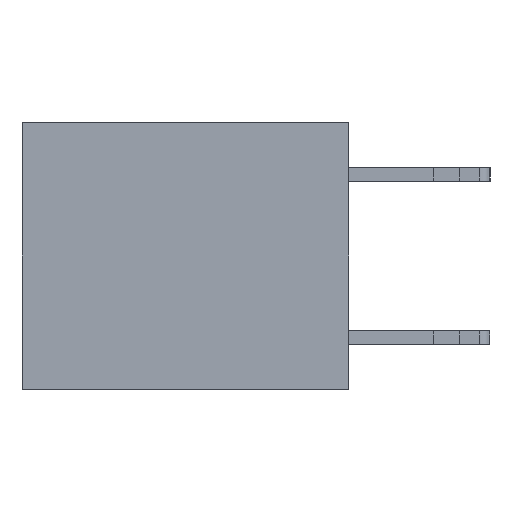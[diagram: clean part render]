
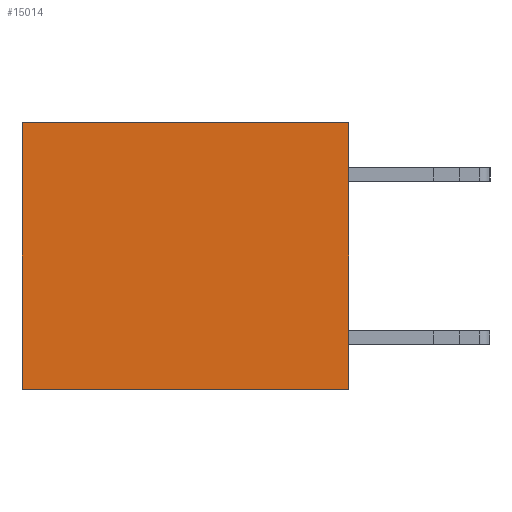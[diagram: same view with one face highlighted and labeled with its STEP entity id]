
A CAD part, left-side view. The second image highlights one B-rep face of the part: STEP entity #15014.
In plain terms, the highlighted planar face has unit normal (-1, 0, 0).
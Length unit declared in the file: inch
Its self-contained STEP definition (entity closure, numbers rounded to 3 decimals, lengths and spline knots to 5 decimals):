
#564 = EDGE_CURVE ( 'NONE', #7860, #4236, #18964, .T. ) ;
#1781 = VECTOR ( 'NONE', #2009, 39.37008 ) ;
#2009 = DIRECTION ( 'NONE',  ( 0., 0., -1. ) ) ;
#2299 = ORIENTED_EDGE ( 'NONE', *, *, #19089, .F. ) ;
#3406 = CARTESIAN_POINT ( 'NONE',  ( 0.3165, 0., 0. ) ) ;
#3525 = CARTESIAN_POINT ( 'NONE',  ( 0.3165, 0., -0.49 ) ) ;
#4236 = VERTEX_POINT ( 'NONE', #15485 ) ;
#5032 = DIRECTION ( 'NONE',  ( 0., 1., 0. ) ) ;
#5411 = CARTESIAN_POINT ( 'NONE',  ( 0.3165, 0., -0.49 ) ) ;
#6189 = VERTEX_POINT ( 'NONE', #16741 ) ;
#6247 = ORIENTED_EDGE ( 'NONE', *, *, #11554, .T. ) ;
#6881 = CARTESIAN_POINT ( 'NONE',  ( 0.3165, 0., -0.49 ) ) ;
#7126 = VERTEX_POINT ( 'NONE', #14093 ) ;
#7707 = LINE ( 'NONE', #3406, #12922 ) ;
#7860 = VERTEX_POINT ( 'NONE', #13289 ) ;
#8170 = VECTOR ( 'NONE', #17472, 39.37008 ) ;
#10008 = DIRECTION ( 'NONE',  ( 1., 0., 0. ) ) ;
#11113 = FACE_OUTER_BOUND ( 'NONE', #14515, .T. ) ;
#11404 = PLANE ( 'NONE',  #16313 ) ;
#11554 = EDGE_CURVE ( 'NONE', #7860, #6189, #7707, .T. ) ;
#12902 = DIRECTION ( 'NONE',  ( 0., 0., -1. ) ) ;
#12922 = VECTOR ( 'NONE', #5032, 39.37008 ) ;
#13289 = CARTESIAN_POINT ( 'NONE',  ( 0.3165, 0., 0. ) ) ;
#13888 = DIRECTION ( 'NONE',  ( 0., 0., -1. ) ) ;
#14093 = CARTESIAN_POINT ( 'NONE',  ( 0.3165, 0.6, -0.49 ) ) ;
#14489 = ORIENTED_EDGE ( 'NONE', *, *, #14897, .T. ) ;
#14515 = EDGE_LOOP ( 'NONE', ( #14489, #2299, #15256, #6247 ) ) ;
#14897 = EDGE_CURVE ( 'NONE', #6189, #7126, #18780, .T. ) ;
#15014 = ADVANCED_FACE ( 'NONE', ( #11113 ), #11404, .F. ) ;
#15017 = LINE ( 'NONE', #5411, #8170 ) ;
#15256 = ORIENTED_EDGE ( 'NONE', *, *, #564, .F. ) ;
#15485 = CARTESIAN_POINT ( 'NONE',  ( 0.3165, 0., -0.49 ) ) ;
#16313 = AXIS2_PLACEMENT_3D ( 'NONE', #6881, #10008, #12902 ) ;
#16634 = VECTOR ( 'NONE', #13888, 39.37008 ) ;
#16741 = CARTESIAN_POINT ( 'NONE',  ( 0.3165, 0.6, 0. ) ) ;
#16826 = CARTESIAN_POINT ( 'NONE',  ( 0.3165, 0.6, -0.49 ) ) ;
#17472 = DIRECTION ( 'NONE',  ( 0., 1., 0. ) ) ;
#18780 = LINE ( 'NONE', #16826, #16634 ) ;
#18964 = LINE ( 'NONE', #3525, #1781 ) ;
#19089 = EDGE_CURVE ( 'NONE', #4236, #7126, #15017, .T. ) ;
